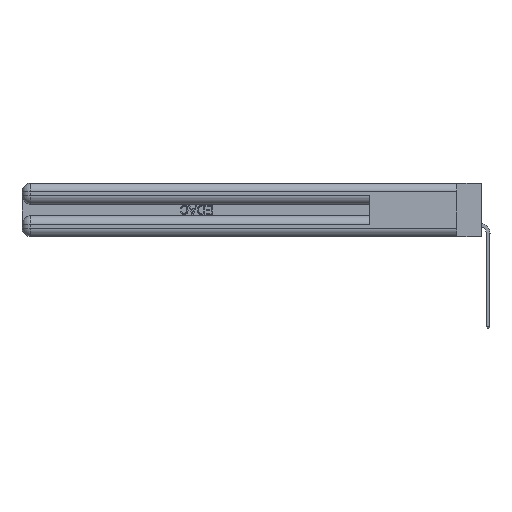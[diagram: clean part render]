
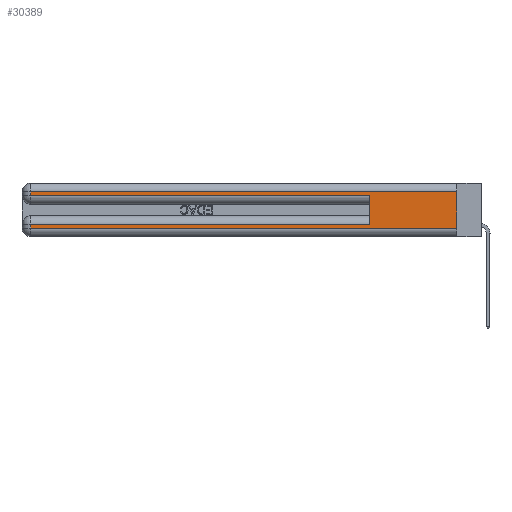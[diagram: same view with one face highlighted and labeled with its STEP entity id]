
A CAD part, left-side view. The second image highlights one B-rep face of the part: STEP entity #30389.
In plain terms, the highlighted planar face has unit normal (-1, 0, 0).
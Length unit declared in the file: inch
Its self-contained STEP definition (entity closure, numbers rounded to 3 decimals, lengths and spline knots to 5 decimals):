
#1366 = CARTESIAN_POINT ( 'NONE',  ( 0., 0., 0.285 ) ) ;
#5369 = EDGE_CURVE ( 'NONE', #26463, #23727, #19470, .T. ) ;
#6543 = ORIENTED_EDGE ( 'NONE', *, *, #22241, .F. ) ;
#6591 = PLANE ( 'NONE',  #13270 ) ;
#7148 = CARTESIAN_POINT ( 'NONE',  ( 0., 0., 0.31 ) ) ;
#7220 = VECTOR ( 'NONE', #19546, 39.37008 ) ;
#9028 = ORIENTED_EDGE ( 'NONE', *, *, #15091, .T. ) ;
#9203 = DIRECTION ( 'NONE',  ( 0., 0., -1. ) ) ;
#9300 = EDGE_CURVE ( 'NONE', #30831, #26463, #12547, .T. ) ;
#9468 = ORIENTED_EDGE ( 'NONE', *, *, #25115, .T. ) ;
#9587 = DIRECTION ( 'NONE',  ( 1., 0., 0. ) ) ;
#10010 = CARTESIAN_POINT ( 'NONE',  ( 0., 2.94, 0.085 ) ) ;
#11045 = CARTESIAN_POINT ( 'NONE',  ( 0., 2.94, 0.37 ) ) ;
#12366 = CARTESIAN_POINT ( 'NONE',  ( 0., 2.94, 0.285 ) ) ;
#12547 = LINE ( 'NONE', #7148, #7220 ) ;
#12801 = VECTOR ( 'NONE', #16910, 39.37008 ) ;
#13270 = AXIS2_PLACEMENT_3D ( 'NONE', #28230, #9587, #9203 ) ;
#13331 = LINE ( 'NONE', #25167, #24463 ) ;
#13606 = ORIENTED_EDGE ( 'NONE', *, *, #5369, .T. ) ;
#14086 = VECTOR ( 'NONE', #28196, 39.37008 ) ;
#14749 = ORIENTED_EDGE ( 'NONE', *, *, #23668, .F. ) ;
#15091 = EDGE_CURVE ( 'NONE', #28793, #24448, #20357, .T. ) ;
#15163 = LINE ( 'NONE', #17524, #30663 ) ;
#16910 = DIRECTION ( 'NONE',  ( 0., -1., 0. ) ) ;
#17233 = DIRECTION ( 'NONE',  ( 0., 0., -1. ) ) ;
#17524 = CARTESIAN_POINT ( 'NONE',  ( 0., 2.94, 0.37 ) ) ;
#17889 = VERTEX_POINT ( 'NONE', #35456 ) ;
#18468 = EDGE_LOOP ( 'NONE', ( #14749, #37796, #13606, #38584, #6543, #9028, #9468, #19923 ) ) ;
#19470 = LINE ( 'NONE', #11045, #22390 ) ;
#19546 = DIRECTION ( 'NONE',  ( 0., 1., 0. ) ) ;
#19923 = ORIENTED_EDGE ( 'NONE', *, *, #21185, .T. ) ;
#20239 = DIRECTION ( 'NONE',  ( 0., -1., 0. ) ) ;
#20357 = LINE ( 'NONE', #25066, #14086 ) ;
#21185 = EDGE_CURVE ( 'NONE', #36984, #17889, #30933, .T. ) ;
#22241 = EDGE_CURVE ( 'NONE', #28793, #22421, #38555, .T. ) ;
#22390 = VECTOR ( 'NONE', #36336, 39.37008 ) ;
#22421 = VERTEX_POINT ( 'NONE', #36015 ) ;
#22562 = CARTESIAN_POINT ( 'NONE',  ( 0., 2.94, 0.31 ) ) ;
#22748 = CARTESIAN_POINT ( 'NONE',  ( 0., 0.6, 0.145 ) ) ;
#23668 = EDGE_CURVE ( 'NONE', #30831, #17889, #13331, .T. ) ;
#23727 = VERTEX_POINT ( 'NONE', #12366 ) ;
#24448 = VERTEX_POINT ( 'NONE', #10010 ) ;
#24463 = VECTOR ( 'NONE', #40107, 39.37008 ) ;
#25066 = CARTESIAN_POINT ( 'NONE',  ( 0., 0., 0.085 ) ) ;
#25115 = EDGE_CURVE ( 'NONE', #24448, #36984, #15163, .T. ) ;
#25167 = CARTESIAN_POINT ( 'NONE',  ( 0., 0., 0.37 ) ) ;
#26463 = VERTEX_POINT ( 'NONE', #22562 ) ;
#27342 = LINE ( 'NONE', #1366, #12801 ) ;
#27438 = CARTESIAN_POINT ( 'NONE',  ( 0., 2.94, 0.06 ) ) ;
#28196 = DIRECTION ( 'NONE',  ( 0., 1., 0. ) ) ;
#28230 = CARTESIAN_POINT ( 'NONE',  ( 0., 0., 0.37 ) ) ;
#28708 = DIRECTION ( 'NONE',  ( 0., 0., 1. ) ) ;
#28793 = VERTEX_POINT ( 'NONE', #37026 ) ;
#29837 = CARTESIAN_POINT ( 'NONE',  ( 0., 0., 0.31 ) ) ;
#29852 = VECTOR ( 'NONE', #28708, 39.37008 ) ;
#30389 = ADVANCED_FACE ( 'NONE', ( #33961 ), #6591, .F. ) ;
#30663 = VECTOR ( 'NONE', #17233, 39.37008 ) ;
#30831 = VERTEX_POINT ( 'NONE', #29837 ) ;
#30933 = LINE ( 'NONE', #32298, #34799 ) ;
#32298 = CARTESIAN_POINT ( 'NONE',  ( 0., 0., 0.06 ) ) ;
#33961 = FACE_OUTER_BOUND ( 'NONE', #18468, .T. ) ;
#34056 = EDGE_CURVE ( 'NONE', #23727, #22421, #27342, .T. ) ;
#34799 = VECTOR ( 'NONE', #20239, 39.37008 ) ;
#35456 = CARTESIAN_POINT ( 'NONE',  ( 0., 0., 0.06 ) ) ;
#36015 = CARTESIAN_POINT ( 'NONE',  ( 0., 0.6, 0.285 ) ) ;
#36336 = DIRECTION ( 'NONE',  ( 0., 0., -1. ) ) ;
#36984 = VERTEX_POINT ( 'NONE', #27438 ) ;
#37026 = CARTESIAN_POINT ( 'NONE',  ( 0., 0.6, 0.085 ) ) ;
#37796 = ORIENTED_EDGE ( 'NONE', *, *, #9300, .T. ) ;
#38555 = LINE ( 'NONE', #22748, #29852 ) ;
#38584 = ORIENTED_EDGE ( 'NONE', *, *, #34056, .T. ) ;
#40107 = DIRECTION ( 'NONE',  ( 0., 0., -1. ) ) ;
